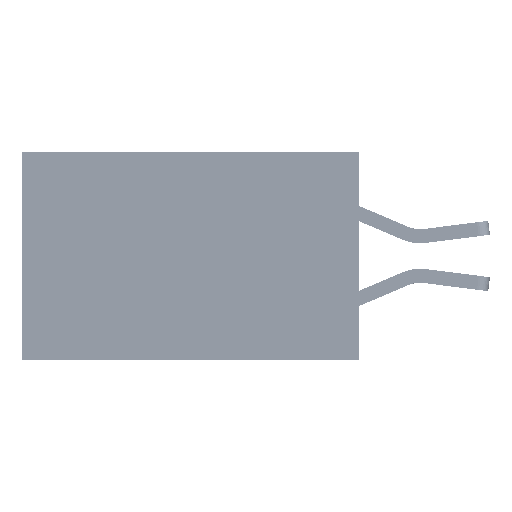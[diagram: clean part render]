
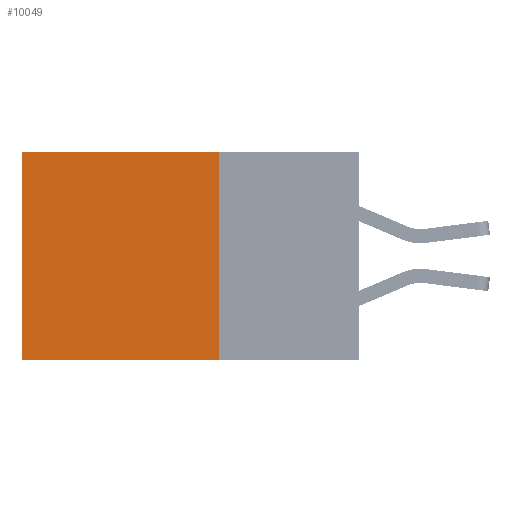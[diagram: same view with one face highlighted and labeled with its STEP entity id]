
A CAD part, left-side view. The second image highlights one B-rep face of the part: STEP entity #10049.
In plain terms, the highlighted planar face has unit normal (-1, 0, 0).
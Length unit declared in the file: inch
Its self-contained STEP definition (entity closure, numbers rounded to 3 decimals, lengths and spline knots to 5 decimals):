
#70 = PLANE ( 'NONE',  #30290 ) ;
#5944 = EDGE_CURVE ( 'NONE', #33844, #36800, #14370, .T. ) ;
#7130 = CARTESIAN_POINT ( 'NONE',  ( 0.2875, 0.25, 0. ) ) ;
#8813 = CARTESIAN_POINT ( 'NONE',  ( 0.2875, 0.25, -0.37 ) ) ;
#10049 = ADVANCED_FACE ( 'NONE', ( #38150 ), #70, .F. ) ;
#11044 = ORIENTED_EDGE ( 'NONE', *, *, #21119, .F. ) ;
#11473 = LINE ( 'NONE', #7130, #23710 ) ;
#11950 = DIRECTION ( 'NONE',  ( 0., 1., 0. ) ) ;
#13396 = VECTOR ( 'NONE', #32577, 39.37008 ) ;
#13628 = VECTOR ( 'NONE', #11950, 39.37008 ) ;
#14370 = LINE ( 'NONE', #32984, #13396 ) ;
#15205 = CARTESIAN_POINT ( 'NONE',  ( 0.2875, 0.25, 0. ) ) ;
#16819 = VERTEX_POINT ( 'NONE', #19027 ) ;
#18791 = CARTESIAN_POINT ( 'NONE',  ( 0.2875, 0.6, 0. ) ) ;
#18890 = CARTESIAN_POINT ( 'NONE',  ( 0.2875, 0.6, 0. ) ) ;
#18966 = ORIENTED_EDGE ( 'NONE', *, *, #5944, .T. ) ;
#19024 = DIRECTION ( 'NONE',  ( 0., 0., -1. ) ) ;
#19027 = CARTESIAN_POINT ( 'NONE',  ( 0.2875, 0.6, -0.37 ) ) ;
#21119 = EDGE_CURVE ( 'NONE', #24635, #16819, #35700, .T. ) ;
#21884 = DIRECTION ( 'NONE',  ( 1., 0., 0. ) ) ;
#23710 = VECTOR ( 'NONE', #25989, 39.37008 ) ;
#24635 = VERTEX_POINT ( 'NONE', #39623 ) ;
#25989 = DIRECTION ( 'NONE',  ( 0., 0., -1. ) ) ;
#27321 = EDGE_CURVE ( 'NONE', #36800, #16819, #35136, .T. ) ;
#30150 = ORIENTED_EDGE ( 'NONE', *, *, #27321, .T. ) ;
#30290 = AXIS2_PLACEMENT_3D ( 'NONE', #15205, #21884, #40377 ) ;
#32577 = DIRECTION ( 'NONE',  ( 0., 1., 0. ) ) ;
#32984 = CARTESIAN_POINT ( 'NONE',  ( 0.2875, 0.25, 0. ) ) ;
#33844 = VERTEX_POINT ( 'NONE', #34323 ) ;
#34323 = CARTESIAN_POINT ( 'NONE',  ( 0.2875, 0.25, 0. ) ) ;
#35136 = LINE ( 'NONE', #18890, #35597 ) ;
#35322 = ORIENTED_EDGE ( 'NONE', *, *, #37042, .F. ) ;
#35597 = VECTOR ( 'NONE', #19024, 39.37008 ) ;
#35700 = LINE ( 'NONE', #8813, #13628 ) ;
#36800 = VERTEX_POINT ( 'NONE', #18791 ) ;
#37042 = EDGE_CURVE ( 'NONE', #33844, #24635, #11473, .T. ) ;
#37711 = EDGE_LOOP ( 'NONE', ( #30150, #11044, #35322, #18966 ) ) ;
#38150 = FACE_OUTER_BOUND ( 'NONE', #37711, .T. ) ;
#39623 = CARTESIAN_POINT ( 'NONE',  ( 0.2875, 0.25, -0.37 ) ) ;
#40377 = DIRECTION ( 'NONE',  ( 0., 0., -1. ) ) ;
